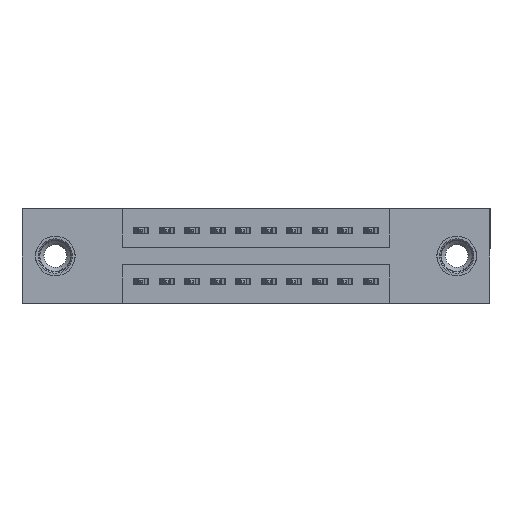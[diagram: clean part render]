
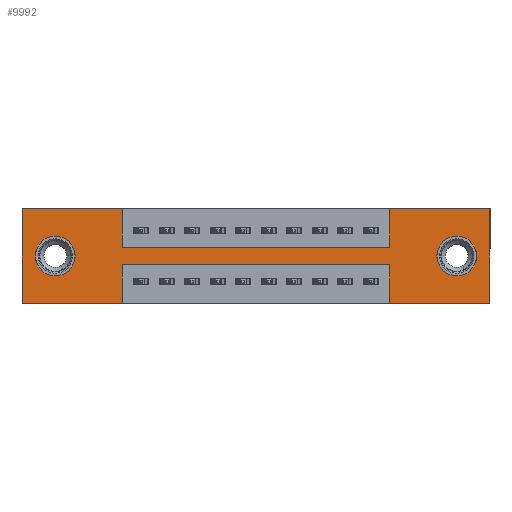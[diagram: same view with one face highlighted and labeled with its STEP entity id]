
A CAD part, front view. The second image highlights one B-rep face of the part: STEP entity #9992.
In plain terms, the highlighted planar face has unit normal (0, -1, 0).
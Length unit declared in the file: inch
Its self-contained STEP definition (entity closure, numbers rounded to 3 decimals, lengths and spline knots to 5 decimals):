
#154 = CARTESIAN_POINT ( 'NONE',  ( 0.3925, 0., -0.37 ) ) ;
#237 = VERTEX_POINT ( 'NONE', #16373 ) ;
#317 = EDGE_CURVE ( 'NONE', #5183, #15258, #6044, .T. ) ;
#429 = DIRECTION ( 'NONE',  ( 0., 0., -1. ) ) ;
#476 = DIRECTION ( 'NONE',  ( 0., 0., 1. ) ) ;
#499 = DIRECTION ( 'NONE',  ( -1., 0., 0. ) ) ;
#850 = CARTESIAN_POINT ( 'NONE',  ( 0., 0., -0.37 ) ) ;
#911 = DIRECTION ( 'NONE',  ( 0., 0., -1. ) ) ;
#968 = DIRECTION ( 'NONE',  ( -1., 0., 0. ) ) ;
#972 = CARTESIAN_POINT ( 'NONE',  ( 1.835, 0., 0. ) ) ;
#1053 = DIRECTION ( 'NONE',  ( -1., 0., 0. ) ) ;
#1097 = LINE ( 'NONE', #14519, #7800 ) ;
#1117 = VECTOR ( 'NONE', #968, 39.37008 ) ;
#1186 = EDGE_CURVE ( 'NONE', #13892, #3384, #1753, .T. ) ;
#1196 = CARTESIAN_POINT ( 'NONE',  ( 1.705, 0., -0.185 ) ) ;
#1206 = CARTESIAN_POINT ( 'NONE',  ( 0.3925, 0., -0.15 ) ) ;
#1255 = CARTESIAN_POINT ( 'NONE',  ( 0., 0., -0.37 ) ) ;
#1291 = EDGE_CURVE ( 'NONE', #237, #2192, #7617, .T. ) ;
#1474 = EDGE_CURVE ( 'NONE', #13569, #6457, #5197, .T. ) ;
#1751 = EDGE_CURVE ( 'NONE', #3384, #5183, #11437, .T. ) ;
#1753 = LINE ( 'NONE', #7112, #5416 ) ;
#1808 = CARTESIAN_POINT ( 'NONE',  ( 0.3925, 0., 0. ) ) ;
#1849 = CARTESIAN_POINT ( 'NONE',  ( 1.4425, 0., -0.15 ) ) ;
#1985 = EDGE_LOOP ( 'NONE', ( #12686, #16049 ) ) ;
#2008 = CARTESIAN_POINT ( 'NONE',  ( 0.13, 0., -0.107 ) ) ;
#2028 = ORIENTED_EDGE ( 'NONE', *, *, #12590, .F. ) ;
#2047 = EDGE_CURVE ( 'NONE', #10172, #15038, #1097, .T. ) ;
#2104 = CARTESIAN_POINT ( 'NONE',  ( 0., 0., 0. ) ) ;
#2192 = VERTEX_POINT ( 'NONE', #2008 ) ;
#2213 = LINE ( 'NONE', #16524, #8858 ) ;
#2241 = DIRECTION ( 'NONE',  ( 1., 0., 0. ) ) ;
#2324 = LINE ( 'NONE', #2104, #14167 ) ;
#2481 = LINE ( 'NONE', #8255, #9111 ) ;
#2593 = EDGE_CURVE ( 'NONE', #5975, #4505, #14616, .T. ) ;
#2679 = CARTESIAN_POINT ( 'NONE',  ( 0., 0., -0.37 ) ) ;
#2901 = VECTOR ( 'NONE', #1053, 39.37008 ) ;
#2953 = EDGE_CURVE ( 'NONE', #15621, #16253, #13836, .T. ) ;
#2974 = CARTESIAN_POINT ( 'NONE',  ( 0.3925, 0., 0. ) ) ;
#3081 = CARTESIAN_POINT ( 'NONE',  ( 0.13, 0., -0.185 ) ) ;
#3161 = CARTESIAN_POINT ( 'NONE',  ( 1.835, 0., -0.37 ) ) ;
#3358 = ORIENTED_EDGE ( 'NONE', *, *, #13157, .F. ) ;
#3384 = VERTEX_POINT ( 'NONE', #5750 ) ;
#3524 = DIRECTION ( 'NONE',  ( 0., 0., 1. ) ) ;
#3574 = ORIENTED_EDGE ( 'NONE', *, *, #1291, .T. ) ;
#3801 = ORIENTED_EDGE ( 'NONE', *, *, #317, .F. ) ;
#3887 = FACE_BOUND ( 'NONE', #1985, .T. ) ;
#4360 = DIRECTION ( 'NONE',  ( 1., 0., 0. ) ) ;
#4469 = DIRECTION ( 'NONE',  ( 0., 0., 1. ) ) ;
#4505 = VERTEX_POINT ( 'NONE', #1206 ) ;
#4801 = CARTESIAN_POINT ( 'NONE',  ( 1.835, 0., 0. ) ) ;
#4841 = ORIENTED_EDGE ( 'NONE', *, *, #16439, .F. ) ;
#5077 = AXIS2_PLACEMENT_3D ( 'NONE', #1196, #16512, #13951 ) ;
#5183 = VERTEX_POINT ( 'NONE', #154 ) ;
#5197 = LINE ( 'NONE', #2679, #1117 ) ;
#5271 = LINE ( 'NONE', #8488, #9527 ) ;
#5416 = VECTOR ( 'NONE', #499, 39.37008 ) ;
#5632 = CARTESIAN_POINT ( 'NONE',  ( 0., 0., -0.37 ) ) ;
#5662 = ORIENTED_EDGE ( 'NONE', *, *, #2047, .F. ) ;
#5750 = CARTESIAN_POINT ( 'NONE',  ( 0.3925, 0., -0.22 ) ) ;
#5789 = CARTESIAN_POINT ( 'NONE',  ( 1.4425, 0., -0.37 ) ) ;
#5818 = CIRCLE ( 'NONE', #16643, 0.078 ) ;
#5975 = VERTEX_POINT ( 'NONE', #1808 ) ;
#6044 = LINE ( 'NONE', #1255, #2901 ) ;
#6070 = ORIENTED_EDGE ( 'NONE', *, *, #6513, .F. ) ;
#6139 = CARTESIAN_POINT ( 'NONE',  ( 1.705, 0., -0.185 ) ) ;
#6261 = VECTOR ( 'NONE', #11281, 39.37008 ) ;
#6457 = VERTEX_POINT ( 'NONE', #5789 ) ;
#6513 = EDGE_CURVE ( 'NONE', #8185, #10172, #5271, .T. ) ;
#6597 = CARTESIAN_POINT ( 'NONE',  ( 0.3925, 0., -0.37 ) ) ;
#7112 = CARTESIAN_POINT ( 'NONE',  ( 0.3925, 0., -0.22 ) ) ;
#7346 = FACE_BOUND ( 'NONE', #14897, .T. ) ;
#7423 = DIRECTION ( 'NONE',  ( 0., 0., -1. ) ) ;
#7465 = ORIENTED_EDGE ( 'NONE', *, *, #1751, .F. ) ;
#7617 = CIRCLE ( 'NONE', #11863, 0.078 ) ;
#7799 = LINE ( 'NONE', #14637, #13829 ) ;
#7800 = VECTOR ( 'NONE', #10946, 39.37008 ) ;
#7817 = CARTESIAN_POINT ( 'NONE',  ( 1.705, 0., -0.263 ) ) ;
#8185 = VERTEX_POINT ( 'NONE', #1849 ) ;
#8247 = VERTEX_POINT ( 'NONE', #15031 ) ;
#8255 = CARTESIAN_POINT ( 'NONE',  ( 0.3925, 0., -0.15 ) ) ;
#8312 = AXIS2_PLACEMENT_3D ( 'NONE', #3081, #12182, #4469 ) ;
#8483 = AXIS2_PLACEMENT_3D ( 'NONE', #850, #8899, #911 ) ;
#8488 = CARTESIAN_POINT ( 'NONE',  ( 1.4425, 0., 0. ) ) ;
#8689 = CIRCLE ( 'NONE', #8312, 0.078 ) ;
#8823 = VECTOR ( 'NONE', #14887, 39.37008 ) ;
#8858 = VECTOR ( 'NONE', #2241, 39.37008 ) ;
#8899 = DIRECTION ( 'NONE',  ( 0., -1., 0. ) ) ;
#9111 = VECTOR ( 'NONE', #4360, 39.37008 ) ;
#9236 = CARTESIAN_POINT ( 'NONE',  ( 1.4425, 0., -0.22 ) ) ;
#9511 = ORIENTED_EDGE ( 'NONE', *, *, #14030, .F. ) ;
#9527 = VECTOR ( 'NONE', #476, 39.37008 ) ;
#9992 = ADVANCED_FACE ( 'NONE', ( #3887, #7346, #14187 ), #15264, .T. ) ;
#10172 = VERTEX_POINT ( 'NONE', #10537 ) ;
#10182 = DIRECTION ( 'NONE',  ( 0., 0., 1. ) ) ;
#10397 = EDGE_CURVE ( 'NONE', #15258, #8247, #2324, .T. ) ;
#10453 = CARTESIAN_POINT ( 'NONE',  ( 1.705, 0., -0.107 ) ) ;
#10537 = CARTESIAN_POINT ( 'NONE',  ( 1.4425, 0., 0. ) ) ;
#10946 = DIRECTION ( 'NONE',  ( 1., 0., 0. ) ) ;
#11033 = CARTESIAN_POINT ( 'NONE',  ( 0.13, 0., -0.185 ) ) ;
#11281 = DIRECTION ( 'NONE',  ( 0., 0., -1. ) ) ;
#11318 = DIRECTION ( 'NONE',  ( 0., 1., 0. ) ) ;
#11437 = LINE ( 'NONE', #6597, #8823 ) ;
#11702 = ORIENTED_EDGE ( 'NONE', *, *, #1474, .F. ) ;
#11863 = AXIS2_PLACEMENT_3D ( 'NONE', #11033, #11318, #10182 ) ;
#12063 = DIRECTION ( 'NONE',  ( 0., 0., 1. ) ) ;
#12182 = DIRECTION ( 'NONE',  ( 0., 1., 0. ) ) ;
#12590 = EDGE_CURVE ( 'NONE', #15038, #13569, #16433, .T. ) ;
#12686 = ORIENTED_EDGE ( 'NONE', *, *, #13647, .T. ) ;
#13157 = EDGE_CURVE ( 'NONE', #8247, #5975, #2213, .T. ) ;
#13325 = ORIENTED_EDGE ( 'NONE', *, *, #2593, .F. ) ;
#13569 = VERTEX_POINT ( 'NONE', #3161 ) ;
#13647 = EDGE_CURVE ( 'NONE', #16253, #15621, #5818, .T. ) ;
#13717 = ORIENTED_EDGE ( 'NONE', *, *, #10397, .F. ) ;
#13815 = VECTOR ( 'NONE', #429, 39.37008 ) ;
#13829 = VECTOR ( 'NONE', #12063, 39.37008 ) ;
#13836 = CIRCLE ( 'NONE', #5077, 0.078 ) ;
#13892 = VERTEX_POINT ( 'NONE', #9236 ) ;
#13951 = DIRECTION ( 'NONE',  ( 0., 0., -1. ) ) ;
#14030 = EDGE_CURVE ( 'NONE', #4505, #8185, #2481, .T. ) ;
#14055 = EDGE_CURVE ( 'NONE', #2192, #237, #8689, .T. ) ;
#14167 = VECTOR ( 'NONE', #3524, 39.37008 ) ;
#14187 = FACE_OUTER_BOUND ( 'NONE', #14663, .T. ) ;
#14307 = ORIENTED_EDGE ( 'NONE', *, *, #1186, .F. ) ;
#14519 = CARTESIAN_POINT ( 'NONE',  ( 0., 0., 0. ) ) ;
#14616 = LINE ( 'NONE', #2974, #13815 ) ;
#14637 = CARTESIAN_POINT ( 'NONE',  ( 1.4425, 0., -0.37 ) ) ;
#14663 = EDGE_LOOP ( 'NONE', ( #7465, #14307, #4841, #11702, #2028, #5662, #6070, #9511, #13325, #3358, #13717, #3801 ) ) ;
#14887 = DIRECTION ( 'NONE',  ( 0., 0., -1. ) ) ;
#14897 = EDGE_LOOP ( 'NONE', ( #16854, #3574 ) ) ;
#15031 = CARTESIAN_POINT ( 'NONE',  ( 0., 0., 0. ) ) ;
#15038 = VERTEX_POINT ( 'NONE', #972 ) ;
#15089 = DIRECTION ( 'NONE',  ( 0., 1., 0. ) ) ;
#15258 = VERTEX_POINT ( 'NONE', #5632 ) ;
#15264 = PLANE ( 'NONE',  #8483 ) ;
#15621 = VERTEX_POINT ( 'NONE', #7817 ) ;
#16049 = ORIENTED_EDGE ( 'NONE', *, *, #2953, .T. ) ;
#16253 = VERTEX_POINT ( 'NONE', #10453 ) ;
#16373 = CARTESIAN_POINT ( 'NONE',  ( 0.13, 0., -0.263 ) ) ;
#16433 = LINE ( 'NONE', #4801, #6261 ) ;
#16439 = EDGE_CURVE ( 'NONE', #6457, #13892, #7799, .T. ) ;
#16512 = DIRECTION ( 'NONE',  ( 0., 1., 0. ) ) ;
#16524 = CARTESIAN_POINT ( 'NONE',  ( 0., 0., 0. ) ) ;
#16643 = AXIS2_PLACEMENT_3D ( 'NONE', #6139, #15089, #7423 ) ;
#16854 = ORIENTED_EDGE ( 'NONE', *, *, #14055, .T. ) ;
